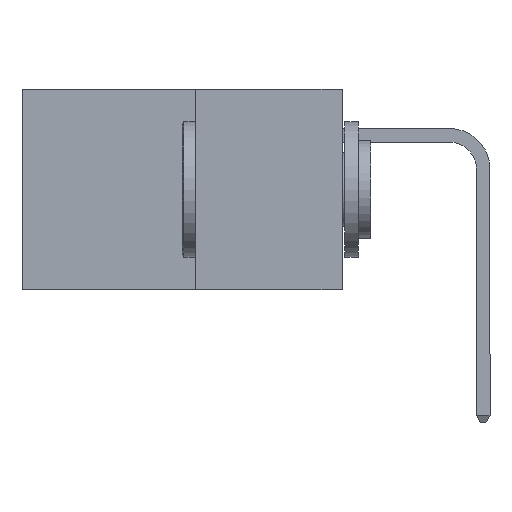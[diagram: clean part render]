
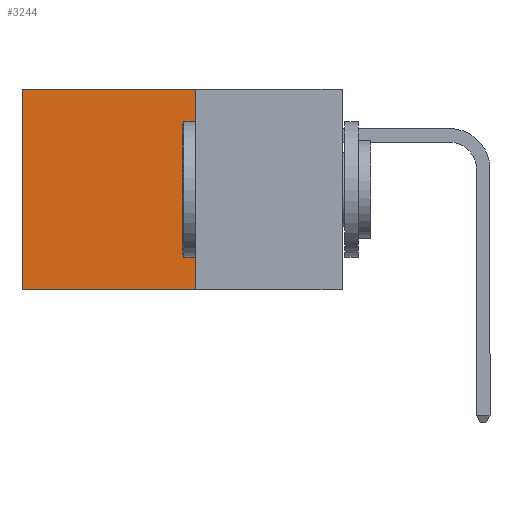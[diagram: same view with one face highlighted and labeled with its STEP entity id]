
A CAD part, left-side view. The second image highlights one B-rep face of the part: STEP entity #3244.
In plain terms, the highlighted planar face has unit normal (-1, 0, 0).
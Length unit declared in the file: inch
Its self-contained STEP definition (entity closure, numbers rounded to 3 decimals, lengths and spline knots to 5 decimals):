
#761 = ORIENTED_EDGE ( 'NONE', *, *, #5536, .F. ) ;
#1056 = AXIS2_PLACEMENT_3D ( 'NONE', #11492, #11229, #6473 ) ;
#1195 = VECTOR ( 'NONE', #9227, 39.37008 ) ;
#1328 = DIRECTION ( 'NONE',  ( 0., 1., 0. ) ) ;
#1451 = CARTESIAN_POINT ( 'NONE',  ( 0.277, 0.27, -0.37 ) ) ;
#1838 = CARTESIAN_POINT ( 'NONE',  ( 0.277, 0.59, -0.37 ) ) ;
#2205 = FACE_OUTER_BOUND ( 'NONE', #5913, .T. ) ;
#2343 = VECTOR ( 'NONE', #9145, 39.37008 ) ;
#2705 = CARTESIAN_POINT ( 'NONE',  ( 0.277, 0.59, 0. ) ) ;
#3244 = ADVANCED_FACE ( 'NONE', ( #2205 ), #6736, .F. ) ;
#3643 = VERTEX_POINT ( 'NONE', #2705 ) ;
#4381 = EDGE_CURVE ( 'NONE', #3643, #10211, #4885, .T. ) ;
#4885 = LINE ( 'NONE', #9048, #2343 ) ;
#5250 = LINE ( 'NONE', #8668, #7949 ) ;
#5536 = EDGE_CURVE ( 'NONE', #7786, #11997, #6562, .T. ) ;
#5640 = EDGE_CURVE ( 'NONE', #7786, #3643, #5250, .T. ) ;
#5823 = VECTOR ( 'NONE', #1328, 39.37008 ) ;
#5913 = EDGE_LOOP ( 'NONE', ( #8383, #6646, #761, #7984 ) ) ;
#6473 = DIRECTION ( 'NONE',  ( 0., 0., -1. ) ) ;
#6562 = LINE ( 'NONE', #9243, #1195 ) ;
#6646 = ORIENTED_EDGE ( 'NONE', *, *, #8613, .F. ) ;
#6718 = CARTESIAN_POINT ( 'NONE',  ( 0.277, 0.27, 0. ) ) ;
#6736 = PLANE ( 'NONE',  #1056 ) ;
#7786 = VERTEX_POINT ( 'NONE', #6718 ) ;
#7949 = VECTOR ( 'NONE', #8654, 39.37008 ) ;
#7984 = ORIENTED_EDGE ( 'NONE', *, *, #5640, .T. ) ;
#8383 = ORIENTED_EDGE ( 'NONE', *, *, #4381, .T. ) ;
#8613 = EDGE_CURVE ( 'NONE', #11997, #10211, #9094, .T. ) ;
#8654 = DIRECTION ( 'NONE',  ( 0., 1., 0. ) ) ;
#8668 = CARTESIAN_POINT ( 'NONE',  ( 0.277, 0.27, 0. ) ) ;
#9048 = CARTESIAN_POINT ( 'NONE',  ( 0.277, 0.59, -0.37 ) ) ;
#9094 = LINE ( 'NONE', #1451, #5823 ) ;
#9145 = DIRECTION ( 'NONE',  ( 0., 0., -1. ) ) ;
#9227 = DIRECTION ( 'NONE',  ( 0., 0., -1. ) ) ;
#9243 = CARTESIAN_POINT ( 'NONE',  ( 0.277, 0.27, -0.37 ) ) ;
#10211 = VERTEX_POINT ( 'NONE', #1838 ) ;
#10848 = CARTESIAN_POINT ( 'NONE',  ( 0.277, 0.27, -0.37 ) ) ;
#11229 = DIRECTION ( 'NONE',  ( 1., 0., 0. ) ) ;
#11492 = CARTESIAN_POINT ( 'NONE',  ( 0.277, 0.27, -0.37 ) ) ;
#11997 = VERTEX_POINT ( 'NONE', #10848 ) ;
